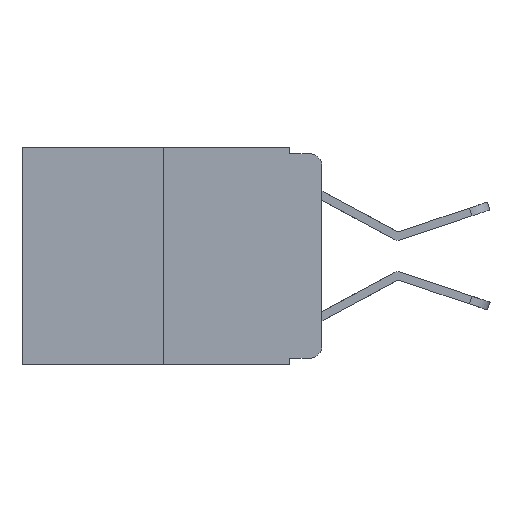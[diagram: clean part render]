
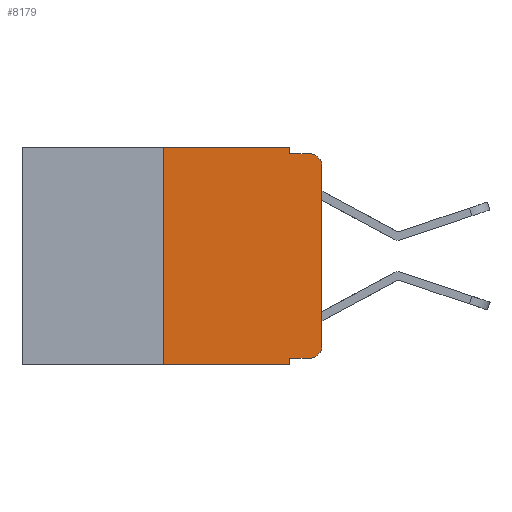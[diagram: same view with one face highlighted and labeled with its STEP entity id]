
A CAD part, left-side view. The second image highlights one B-rep face of the part: STEP entity #8179.
In plain terms, the highlighted planar face has unit normal (-1, 0, 0).
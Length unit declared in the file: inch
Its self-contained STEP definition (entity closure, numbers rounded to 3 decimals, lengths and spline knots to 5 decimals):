
#68 = LINE ( 'NONE', #6920, #11698 ) ;
#408 = ORIENTED_EDGE ( 'NONE', *, *, #7262, .F. ) ;
#1019 = DIRECTION ( 'NONE',  ( 0., 0., -1. ) ) ;
#1050 = FACE_OUTER_BOUND ( 'NONE', #3901, .T. ) ;
#1398 = LINE ( 'NONE', #10156, #8245 ) ;
#1417 = LINE ( 'NONE', #7347, #4612 ) ;
#1517 = DIRECTION ( 'NONE',  ( 0., -1., 0. ) ) ;
#1766 = DIRECTION ( 'NONE',  ( 0., -1., 0. ) ) ;
#1942 = DIRECTION ( 'NONE',  ( 0., 0., -1. ) ) ;
#2119 = VERTEX_POINT ( 'NONE', #4554 ) ;
#2316 = CARTESIAN_POINT ( 'NONE',  ( 0., 0.473, -0.343 ) ) ;
#2756 = ORIENTED_EDGE ( 'NONE', *, *, #9881, .T. ) ;
#2906 = CARTESIAN_POINT ( 'NONE',  ( 0., 0.051, -0.343 ) ) ;
#3087 = LINE ( 'NONE', #9795, #11597 ) ;
#3133 = LINE ( 'NONE', #2316, #10530 ) ;
#3181 = AXIS2_PLACEMENT_3D ( 'NONE', #10868, #3957, #7737 ) ;
#3233 = VERTEX_POINT ( 'NONE', #3279 ) ;
#3279 = CARTESIAN_POINT ( 'NONE',  ( 0., 0.02, -0.333 ) ) ;
#3327 = CARTESIAN_POINT ( 'NONE',  ( 0., 0., -0.03 ) ) ;
#3637 = VECTOR ( 'NONE', #11152, 39.37008 ) ;
#3697 = CARTESIAN_POINT ( 'NONE',  ( 0., 0., -0.313 ) ) ;
#3776 = VERTEX_POINT ( 'NONE', #3327 ) ;
#3807 = ORIENTED_EDGE ( 'NONE', *, *, #9011, .F. ) ;
#3818 = EDGE_CURVE ( 'NONE', #11994, #7932, #4543, .T. ) ;
#3833 = DIRECTION ( 'NONE',  ( 0., 0., -1. ) ) ;
#3884 = VERTEX_POINT ( 'NONE', #10702 ) ;
#3901 = EDGE_LOOP ( 'NONE', ( #2756, #10576, #4110, #408, #3807, #8070, #6072, #7464, #5819, #6364 ) ) ;
#3909 = VERTEX_POINT ( 'NONE', #8681 ) ;
#3957 = DIRECTION ( 'NONE',  ( -1., 0., 0. ) ) ;
#4103 = CIRCLE ( 'NONE', #6760, 0.02 ) ;
#4110 = ORIENTED_EDGE ( 'NONE', *, *, #8691, .F. ) ;
#4202 = CIRCLE ( 'NONE', #3181, 0.02 ) ;
#4255 = VERTEX_POINT ( 'NONE', #3697 ) ;
#4404 = DIRECTION ( 'NONE',  ( 1., 0., 0. ) ) ;
#4543 = LINE ( 'NONE', #12151, #3637 ) ;
#4554 = CARTESIAN_POINT ( 'NONE',  ( 0., 0.051, -0.01 ) ) ;
#4612 = VECTOR ( 'NONE', #5233, 39.37008 ) ;
#4794 = DIRECTION ( 'NONE',  ( -1., 0., 0. ) ) ;
#5233 = DIRECTION ( 'NONE',  ( 0., -1., 0. ) ) ;
#5806 = CARTESIAN_POINT ( 'NONE',  ( 0., 0.02, -0.313 ) ) ;
#5819 = ORIENTED_EDGE ( 'NONE', *, *, #6347, .T. ) ;
#6072 = ORIENTED_EDGE ( 'NONE', *, *, #7869, .T. ) ;
#6205 = DIRECTION ( 'NONE',  ( 0., -1., 0. ) ) ;
#6347 = EDGE_CURVE ( 'NONE', #8847, #3233, #68, .T. ) ;
#6364 = ORIENTED_EDGE ( 'NONE', *, *, #10078, .T. ) ;
#6692 = DIRECTION ( 'NONE',  ( 0., 0., -1. ) ) ;
#6727 = EDGE_CURVE ( 'NONE', #3776, #3909, #4202, .T. ) ;
#6760 = AXIS2_PLACEMENT_3D ( 'NONE', #5806, #4794, #3833 ) ;
#6891 = CARTESIAN_POINT ( 'NONE',  ( 0., 0.25, -0.343 ) ) ;
#6920 = CARTESIAN_POINT ( 'NONE',  ( 0., 0.051, -0.333 ) ) ;
#7009 = CARTESIAN_POINT ( 'NONE',  ( 0., 0.051, -0.333 ) ) ;
#7042 = CARTESIAN_POINT ( 'NONE',  ( 0., 0.25, 0. ) ) ;
#7069 = VECTOR ( 'NONE', #7298, 39.37008 ) ;
#7262 = EDGE_CURVE ( 'NONE', #3884, #2119, #3087, .T. ) ;
#7272 = VERTEX_POINT ( 'NONE', #2906 ) ;
#7298 = DIRECTION ( 'NONE',  ( 0., 0., 1. ) ) ;
#7347 = CARTESIAN_POINT ( 'NONE',  ( 0., 0.473, 0. ) ) ;
#7464 = ORIENTED_EDGE ( 'NONE', *, *, #9155, .F. ) ;
#7601 = CARTESIAN_POINT ( 'NONE',  ( 0., 0.051, 0. ) ) ;
#7734 = AXIS2_PLACEMENT_3D ( 'NONE', #10630, #4404, #1942 ) ;
#7737 = DIRECTION ( 'NONE',  ( 0., 0., -1. ) ) ;
#7869 = EDGE_CURVE ( 'NONE', #11994, #7272, #3133, .T. ) ;
#7932 = VERTEX_POINT ( 'NONE', #7042 ) ;
#8070 = ORIENTED_EDGE ( 'NONE', *, *, #3818, .F. ) ;
#8179 = ADVANCED_FACE ( 'NONE', ( #1050 ), #9827, .F. ) ;
#8245 = VECTOR ( 'NONE', #1517, 39.37008 ) ;
#8681 = CARTESIAN_POINT ( 'NONE',  ( 0., 0.02, -0.01 ) ) ;
#8691 = EDGE_CURVE ( 'NONE', #2119, #3909, #1398, .T. ) ;
#8847 = VERTEX_POINT ( 'NONE', #7009 ) ;
#9011 = EDGE_CURVE ( 'NONE', #7932, #3884, #1417, .T. ) ;
#9155 = EDGE_CURVE ( 'NONE', #8847, #7272, #12431, .T. ) ;
#9795 = CARTESIAN_POINT ( 'NONE',  ( 0., 0.051, 0. ) ) ;
#9827 = PLANE ( 'NONE',  #7734 ) ;
#9881 = EDGE_CURVE ( 'NONE', #4255, #3776, #10308, .T. ) ;
#10078 = EDGE_CURVE ( 'NONE', #3233, #4255, #4103, .T. ) ;
#10127 = CARTESIAN_POINT ( 'NONE',  ( 0., 0., 0. ) ) ;
#10156 = CARTESIAN_POINT ( 'NONE',  ( 0., 0.051, -0.01 ) ) ;
#10308 = LINE ( 'NONE', #10127, #7069 ) ;
#10530 = VECTOR ( 'NONE', #6205, 39.37008 ) ;
#10576 = ORIENTED_EDGE ( 'NONE', *, *, #6727, .T. ) ;
#10630 = CARTESIAN_POINT ( 'NONE',  ( 0., 0.473, 0. ) ) ;
#10702 = CARTESIAN_POINT ( 'NONE',  ( 0., 0.051, 0. ) ) ;
#10868 = CARTESIAN_POINT ( 'NONE',  ( 0., 0.02, -0.03 ) ) ;
#11152 = DIRECTION ( 'NONE',  ( 0., 0., 1. ) ) ;
#11597 = VECTOR ( 'NONE', #1019, 39.37008 ) ;
#11698 = VECTOR ( 'NONE', #1766, 39.37008 ) ;
#11994 = VERTEX_POINT ( 'NONE', #6891 ) ;
#12007 = VECTOR ( 'NONE', #6692, 39.37008 ) ;
#12151 = CARTESIAN_POINT ( 'NONE',  ( 0., 0.25, 0. ) ) ;
#12431 = LINE ( 'NONE', #7601, #12007 ) ;
